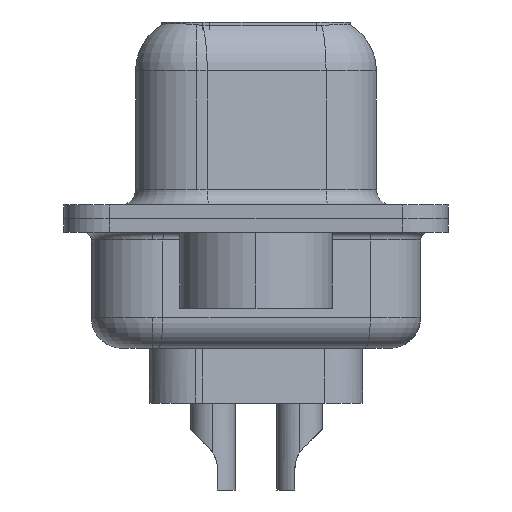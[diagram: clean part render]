
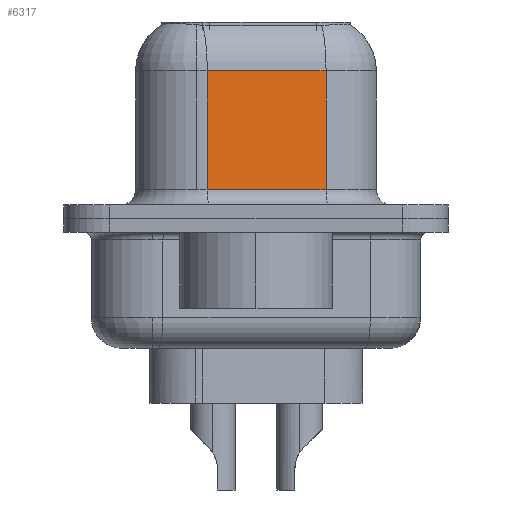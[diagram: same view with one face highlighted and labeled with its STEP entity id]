
A CAD part, left-side view. The second image highlights one B-rep face of the part: STEP entity #6317.
In plain terms, the highlighted planar face has unit normal (-0.985, -0.174, 0).
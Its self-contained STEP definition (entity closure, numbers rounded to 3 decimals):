
#741 = DIRECTION ( 'NONE',  ( 0.985, 0.174, 0. ) ) ;
#1082 = VERTEX_POINT ( 'NONE', #13004 ) ;
#1268 = VECTOR ( 'NONE', #23380, 1000. ) ;
#1892 = CARTESIAN_POINT ( 'NONE',  ( 4.35, 1.603, 6.6 ) ) ;
#1896 = EDGE_CURVE ( 'NONE', #8151, #20026, #16320, .T. ) ;
#2859 = ORIENTED_EDGE ( 'NONE', *, *, #23777, .T. ) ;
#2943 = CARTESIAN_POINT ( 'NONE',  ( 5.038, -2.297, 6.6 ) ) ;
#3190 = EDGE_CURVE ( 'NONE', #9535, #1082, #19405, .T. ) ;
#3324 = FACE_OUTER_BOUND ( 'NONE', #21560, .T. ) ;
#4032 = LINE ( 'NONE', #23098, #7784 ) ;
#5392 = CARTESIAN_POINT ( 'NONE',  ( 5.038, -2.297, 0.95 ) ) ;
#6317 = ADVANCED_FACE ( 'NONE', ( #3324 ), #24683, .F. ) ;
#7296 = DIRECTION ( 'NONE',  ( 0.174, -0.985, 0. ) ) ;
#7430 = VECTOR ( 'NONE', #19034, 1000. ) ;
#7757 = DIRECTION ( 'NONE',  ( -0.174, 0.985, 0. ) ) ;
#7784 = VECTOR ( 'NONE', #7757, 1000. ) ;
#8151 = VERTEX_POINT ( 'NONE', #14812 ) ;
#8375 = VECTOR ( 'NONE', #7296, 1000. ) ;
#8996 = AXIS2_PLACEMENT_3D ( 'NONE', #2943, #741, #13065 ) ;
#9535 = VERTEX_POINT ( 'NONE', #12595 ) ;
#10577 = ORIENTED_EDGE ( 'NONE', *, *, #17311, .T. ) ;
#12595 = CARTESIAN_POINT ( 'NONE',  ( 4.35, 1.603, 4.85 ) ) ;
#13004 = CARTESIAN_POINT ( 'NONE',  ( 4.35, 1.603, 0.95 ) ) ;
#13065 = DIRECTION ( 'NONE',  ( -0.174, 0.985, 0. ) ) ;
#14812 = CARTESIAN_POINT ( 'NONE',  ( 5.038, -2.297, 4.85 ) ) ;
#15686 = ORIENTED_EDGE ( 'NONE', *, *, #3190, .T. ) ;
#16320 = LINE ( 'NONE', #24167, #1268 ) ;
#17311 = EDGE_CURVE ( 'NONE', #1082, #20026, #22884, .T. ) ;
#17438 = CARTESIAN_POINT ( 'NONE',  ( 5.038, -2.297, 0.95 ) ) ;
#19034 = DIRECTION ( 'NONE',  ( 0., 0., -1. ) ) ;
#19405 = LINE ( 'NONE', #1892, #7430 ) ;
#20026 = VERTEX_POINT ( 'NONE', #17438 ) ;
#21560 = EDGE_LOOP ( 'NONE', ( #23648, #2859, #15686, #10577 ) ) ;
#22884 = LINE ( 'NONE', #5392, #8375 ) ;
#23098 = CARTESIAN_POINT ( 'NONE',  ( 5.038, -2.297, 4.85 ) ) ;
#23380 = DIRECTION ( 'NONE',  ( 0., 0., -1. ) ) ;
#23648 = ORIENTED_EDGE ( 'NONE', *, *, #1896, .F. ) ;
#23777 = EDGE_CURVE ( 'NONE', #8151, #9535, #4032, .T. ) ;
#24167 = CARTESIAN_POINT ( 'NONE',  ( 5.038, -2.297, 6.6 ) ) ;
#24683 = PLANE ( 'NONE',  #8996 ) ;
